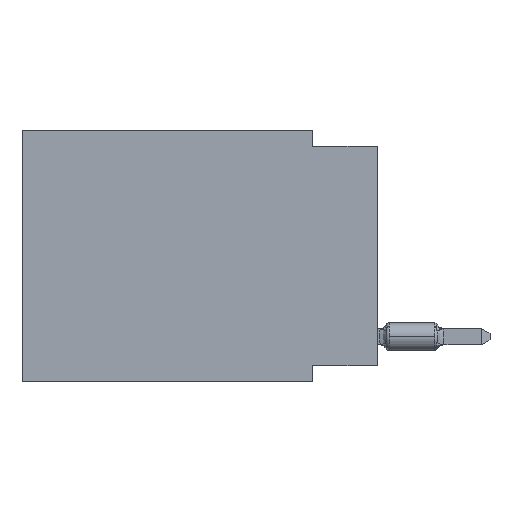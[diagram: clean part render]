
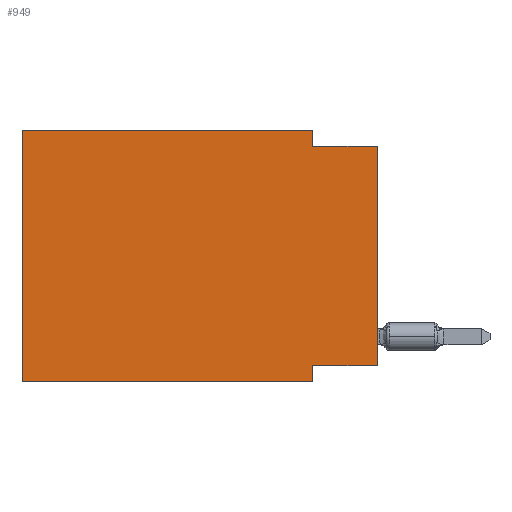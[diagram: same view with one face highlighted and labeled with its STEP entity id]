
A CAD part, left-side view. The second image highlights one B-rep face of the part: STEP entity #949.
In plain terms, the highlighted planar face has unit normal (-1, 0, 0).
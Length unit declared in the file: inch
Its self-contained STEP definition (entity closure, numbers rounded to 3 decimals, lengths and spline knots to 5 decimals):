
#66 = DIRECTION ( 'NONE',  ( 0., 1., 0. ) ) ;
#495 = EDGE_LOOP ( 'NONE', ( #5018, #6837, #12451, #9684, #14036, #4290, #1416, #9843 ) ) ;
#949 = ADVANCED_FACE ( 'NONE', ( #3348 ), #7532, .F. ) ;
#952 = DIRECTION ( 'NONE',  ( 0., -1., 0. ) ) ;
#972 = CARTESIAN_POINT ( 'NONE',  ( 0., 0.1, 0. ) ) ;
#1255 = CARTESIAN_POINT ( 'NONE',  ( 0., 0.55, 0. ) ) ;
#1416 = ORIENTED_EDGE ( 'NONE', *, *, #8745, .F. ) ;
#1536 = LINE ( 'NONE', #9155, #2924 ) ;
#1539 = VECTOR ( 'NONE', #66, 39.37008 ) ;
#1955 = LINE ( 'NONE', #6470, #5219 ) ;
#2364 = CARTESIAN_POINT ( 'NONE',  ( 0., 0.1, -0.025 ) ) ;
#2667 = VECTOR ( 'NONE', #6349, 39.37008 ) ;
#2924 = VECTOR ( 'NONE', #9221, 39.37008 ) ;
#3348 = FACE_OUTER_BOUND ( 'NONE', #495, .T. ) ;
#3860 = CARTESIAN_POINT ( 'NONE',  ( 0., 0.1, -0.365 ) ) ;
#3923 = EDGE_CURVE ( 'NONE', #7440, #9566, #4475, .T. ) ;
#4112 = LINE ( 'NONE', #11745, #2667 ) ;
#4290 = ORIENTED_EDGE ( 'NONE', *, *, #4743, .T. ) ;
#4475 = LINE ( 'NONE', #1255, #6625 ) ;
#4570 = VERTEX_POINT ( 'NONE', #12908 ) ;
#4743 = EDGE_CURVE ( 'NONE', #6638, #12113, #10110, .T. ) ;
#5018 = ORIENTED_EDGE ( 'NONE', *, *, #13099, .T. ) ;
#5219 = VECTOR ( 'NONE', #952, 39.37008 ) ;
#5360 = DIRECTION ( 'NONE',  ( 0., 0., -1. ) ) ;
#5480 = DIRECTION ( 'NONE',  ( 0., 0., -1. ) ) ;
#5724 = CARTESIAN_POINT ( 'NONE',  ( 0., 0.55, -0.39 ) ) ;
#6313 = AXIS2_PLACEMENT_3D ( 'NONE', #14185, #10846, #10774 ) ;
#6349 = DIRECTION ( 'NONE',  ( 0., 0., 1. ) ) ;
#6470 = CARTESIAN_POINT ( 'NONE',  ( 0., 0., -0.025 ) ) ;
#6622 = CARTESIAN_POINT ( 'NONE',  ( 0., 0.1, 0. ) ) ;
#6625 = VECTOR ( 'NONE', #12310, 39.37008 ) ;
#6638 = VERTEX_POINT ( 'NONE', #11809 ) ;
#6728 = DIRECTION ( 'NONE',  ( 0., -1., 0. ) ) ;
#6837 = ORIENTED_EDGE ( 'NONE', *, *, #11775, .F. ) ;
#7440 = VERTEX_POINT ( 'NONE', #11144 ) ;
#7460 = CARTESIAN_POINT ( 'NONE',  ( 0., 0.1, -0.39 ) ) ;
#7532 = PLANE ( 'NONE',  #6313 ) ;
#7540 = CARTESIAN_POINT ( 'NONE',  ( 0., 0.1, -0.39 ) ) ;
#7674 = CARTESIAN_POINT ( 'NONE',  ( 0., 0., -0.365 ) ) ;
#8745 = EDGE_CURVE ( 'NONE', #10771, #12113, #12912, .T. ) ;
#8999 = VERTEX_POINT ( 'NONE', #2364 ) ;
#9155 = CARTESIAN_POINT ( 'NONE',  ( 0., 0., 0. ) ) ;
#9221 = DIRECTION ( 'NONE',  ( 0., 0., 1. ) ) ;
#9566 = VERTEX_POINT ( 'NONE', #6622 ) ;
#9684 = ORIENTED_EDGE ( 'NONE', *, *, #3923, .F. ) ;
#9843 = ORIENTED_EDGE ( 'NONE', *, *, #12303, .F. ) ;
#10110 = LINE ( 'NONE', #5724, #13732 ) ;
#10771 = VERTEX_POINT ( 'NONE', #3860 ) ;
#10774 = DIRECTION ( 'NONE',  ( 0., 0., -1. ) ) ;
#10846 = DIRECTION ( 'NONE',  ( 1., 0., 0. ) ) ;
#11144 = CARTESIAN_POINT ( 'NONE',  ( 0., 0.55, 0. ) ) ;
#11500 = VERTEX_POINT ( 'NONE', #12106 ) ;
#11745 = CARTESIAN_POINT ( 'NONE',  ( 0., 0.55, 0. ) ) ;
#11775 = EDGE_CURVE ( 'NONE', #8999, #4570, #1955, .T. ) ;
#11809 = CARTESIAN_POINT ( 'NONE',  ( 0., 0.55, -0.39 ) ) ;
#12019 = LINE ( 'NONE', #972, #12090 ) ;
#12090 = VECTOR ( 'NONE', #5480, 39.37008 ) ;
#12106 = CARTESIAN_POINT ( 'NONE',  ( 0., 0., -0.365 ) ) ;
#12113 = VERTEX_POINT ( 'NONE', #7540 ) ;
#12303 = EDGE_CURVE ( 'NONE', #11500, #10771, #13128, .T. ) ;
#12310 = DIRECTION ( 'NONE',  ( 0., -1., 0. ) ) ;
#12451 = ORIENTED_EDGE ( 'NONE', *, *, #13004, .F. ) ;
#12908 = CARTESIAN_POINT ( 'NONE',  ( 0., 0., -0.025 ) ) ;
#12912 = LINE ( 'NONE', #7460, #13414 ) ;
#13004 = EDGE_CURVE ( 'NONE', #9566, #8999, #12019, .T. ) ;
#13099 = EDGE_CURVE ( 'NONE', #11500, #4570, #1536, .T. ) ;
#13128 = LINE ( 'NONE', #7674, #1539 ) ;
#13414 = VECTOR ( 'NONE', #5360, 39.37008 ) ;
#13732 = VECTOR ( 'NONE', #6728, 39.37008 ) ;
#14036 = ORIENTED_EDGE ( 'NONE', *, *, #14150, .F. ) ;
#14150 = EDGE_CURVE ( 'NONE', #6638, #7440, #4112, .T. ) ;
#14185 = CARTESIAN_POINT ( 'NONE',  ( 0., 0.55, 0. ) ) ;
